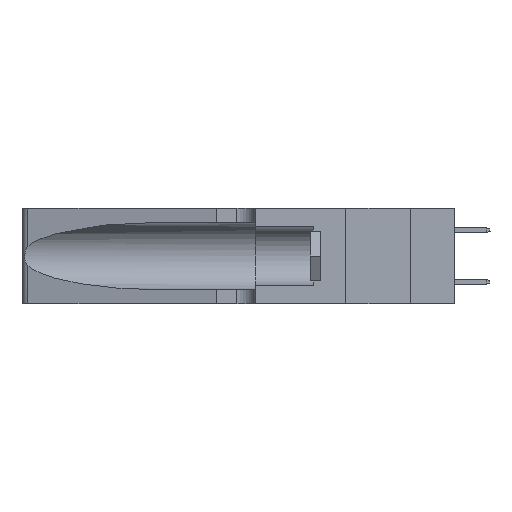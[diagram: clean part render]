
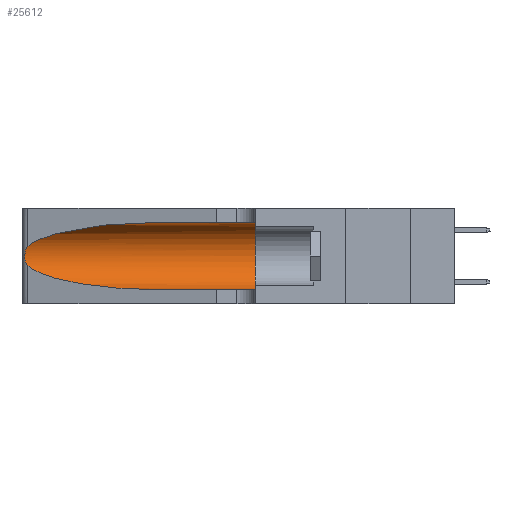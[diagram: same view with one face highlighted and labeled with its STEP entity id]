
A CAD part, left-side view. The second image highlights one B-rep face of the part: STEP entity #25612.
In plain terms, the highlighted cylindrical face has radius 3.308 mm (diameter 6.617 mm), a partial arc.
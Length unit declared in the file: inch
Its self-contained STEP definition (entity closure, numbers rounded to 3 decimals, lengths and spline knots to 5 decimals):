
#1521 = CARTESIAN_POINT ( 'NONE',  ( 0.26075, 1.23896, 0.19203 ) ) ;
#2905 = DIRECTION ( 'NONE',  ( 0., -1., 0. ) ) ;
#3774 = CARTESIAN_POINT ( 'NONE',  ( 0.25787, 1.23484, 0.2124 ) ) ;
#4326 = VERTEX_POINT ( 'NONE', #22807 ) ;
#4682 = CARTESIAN_POINT ( 'NONE',  ( 0.18966, 0.96281, 0.05475 ) ) ;
#4904 = CIRCLE ( 'NONE', #15176, 0.13025 ) ;
#5823 = VERTEX_POINT ( 'NONE', #24263 ) ;
#6220 = LINE ( 'NONE', #22452, #6288 ) ;
#6288 = VECTOR ( 'NONE', #8792, 39.37008 ) ;
#7240 = CYLINDRICAL_SURFACE ( 'NONE', #15799, 0.13025 ) ;
#7782 = B_SPLINE_CURVE_WITH_KNOTS ( 'NONE', 3,
 ( #24721, #13415, #13701, #3774, #8774, #27595, #1521, #20250, #27433, #15850, #29593, #20553, #20094, #10948 ),
 .UNSPECIFIED., .F., .F.,
 ( 4, 2, 2, 2, 2, 2, 4 ),
 ( 0., 0.00027, 0.00053, 0.00107, 0.0016, 0.00187, 0.00214 ),
 .UNSPECIFIED. ) ;
#8774 = CARTESIAN_POINT ( 'NONE',  ( 0.25854, 1.2359, 0.20912 ) ) ;
#8792 = DIRECTION ( 'NONE',  ( 0., -1., 0. ) ) ;
#9292 = CARTESIAN_POINT ( 'NONE',  ( 0.1305, 1.61858, 0.31525 ) ) ;
#9365 = CARTESIAN_POINT ( 'NONE',  ( 0.1305, 1.61858, 0.185 ) ) ;
#10886 =( BOUNDED_CURVE ( )  B_SPLINE_CURVE ( 3, ( #14642, #14173, #16597, #23944 ),
 .UNSPECIFIED., .F., .T. ) 
 B_SPLINE_CURVE_WITH_KNOTS ( ( 4, 4 ),
 ( 1.5708, 2.84003 ),
 .UNSPECIFIED. ) 
 CURVE ( )  GEOMETRIC_REPRESENTATION_ITEM ( )  RATIONAL_B_SPLINE_CURVE ( ( 1., 0.87, 0.87, 1. ) ) 
 REPRESENTATION_ITEM ( '' )  );
#10948 = CARTESIAN_POINT ( 'NONE',  ( 0.25487, 1.22718, 0.14631 ) ) ;
#11378 = EDGE_CURVE ( 'NONE', #4326, #26176, #6220, .T. ) ;
#11673 = FACE_OUTER_BOUND ( 'NONE', #22206, .T. ) ;
#11925 = EDGE_CURVE ( 'NONE', #13277, #26176, #4904, .T. ) ;
#12042 = CARTESIAN_POINT ( 'NONE',  ( 0.1305, 0.72297, 0.31525 ) ) ;
#12053 = LINE ( 'NONE', #9292, #14720 ) ;
#12310 = VERTEX_POINT ( 'NONE', #16334 ) ;
#12837 =( BOUNDED_CURVE ( )  B_SPLINE_CURVE ( 3, ( #13420, #25627, #4682, #14018 ),
 .UNSPECIFIED., .F., .T. ) 
 B_SPLINE_CURVE_WITH_KNOTS ( ( 4, 4 ),
 ( 3.44316, 4.71239 ),
 .UNSPECIFIED. ) 
 CURVE ( )  GEOMETRIC_REPRESENTATION_ITEM ( )  RATIONAL_B_SPLINE_CURVE ( ( 1., 0.87, 0.87, 1. ) ) 
 REPRESENTATION_ITEM ( '' )  );
#12985 = CARTESIAN_POINT ( 'NONE',  ( 0.1305, 0.35, 0.31525 ) ) ;
#13277 = VERTEX_POINT ( 'NONE', #12985 ) ;
#13415 = CARTESIAN_POINT ( 'NONE',  ( 0.25555, 1.22994, 0.2215 ) ) ;
#13420 = CARTESIAN_POINT ( 'NONE',  ( 0.25487, 1.22718, 0.14631 ) ) ;
#13436 = CARTESIAN_POINT ( 'NONE',  ( 0.1305, 0.35, 0.05475 ) ) ;
#13701 = CARTESIAN_POINT ( 'NONE',  ( 0.25639, 1.23184, 0.21858 ) ) ;
#14018 = CARTESIAN_POINT ( 'NONE',  ( 0.1305, 0.72297, 0.05475 ) ) ;
#14173 = CARTESIAN_POINT ( 'NONE',  ( 0.18966, 0.96281, 0.31525 ) ) ;
#14642 = CARTESIAN_POINT ( 'NONE',  ( 0.1305, 0.72297, 0.31525 ) ) ;
#14720 = VECTOR ( 'NONE', #2905, 39.37008 ) ;
#15176 = AXIS2_PLACEMENT_3D ( 'NONE', #24826, #27539, #15201 ) ;
#15201 = DIRECTION ( 'NONE',  ( 0., 0., 1. ) ) ;
#15799 = AXIS2_PLACEMENT_3D ( 'NONE', #9365, #25883, #20974 ) ;
#15850 = CARTESIAN_POINT ( 'NONE',  ( 0.25856, 1.23593, 0.16098 ) ) ;
#16172 = EDGE_CURVE ( 'NONE', #26030, #5823, #10886, .T. ) ;
#16334 = CARTESIAN_POINT ( 'NONE',  ( 0.25487, 1.22718, 0.14631 ) ) ;
#16597 = CARTESIAN_POINT ( 'NONE',  ( 0.2373, 1.15595, 0.28018 ) ) ;
#19498 = ORIENTED_EDGE ( 'NONE', *, *, #11925, .F. ) ;
#19509 = ORIENTED_EDGE ( 'NONE', *, *, #22715, .F. ) ;
#20094 = CARTESIAN_POINT ( 'NONE',  ( 0.25555, 1.22993, 0.14849 ) ) ;
#20250 = CARTESIAN_POINT ( 'NONE',  ( 0.26075, 1.23896, 0.178 ) ) ;
#20553 = CARTESIAN_POINT ( 'NONE',  ( 0.25639, 1.23186, 0.15144 ) ) ;
#20974 = DIRECTION ( 'NONE',  ( 0., 0., -1. ) ) ;
#21013 = EDGE_CURVE ( 'NONE', #5823, #12310, #7782, .T. ) ;
#22206 = EDGE_LOOP ( 'NONE', ( #23520, #28682, #24852, #24189, #19498, #19509 ) ) ;
#22452 = CARTESIAN_POINT ( 'NONE',  ( 0.1305, 1.61858, 0.05475 ) ) ;
#22715 = EDGE_CURVE ( 'NONE', #26030, #13277, #12053, .T. ) ;
#22807 = CARTESIAN_POINT ( 'NONE',  ( 0.1305, 0.72297, 0.05475 ) ) ;
#23520 = ORIENTED_EDGE ( 'NONE', *, *, #16172, .T. ) ;
#23801 = EDGE_CURVE ( 'NONE', #12310, #4326, #12837, .T. ) ;
#23944 = CARTESIAN_POINT ( 'NONE',  ( 0.25487, 1.22718, 0.22369 ) ) ;
#24189 = ORIENTED_EDGE ( 'NONE', *, *, #11378, .T. ) ;
#24263 = CARTESIAN_POINT ( 'NONE',  ( 0.25487, 1.22718, 0.22369 ) ) ;
#24721 = CARTESIAN_POINT ( 'NONE',  ( 0.25487, 1.22718, 0.22369 ) ) ;
#24826 = CARTESIAN_POINT ( 'NONE',  ( 0.1305, 0.35, 0.185 ) ) ;
#24852 = ORIENTED_EDGE ( 'NONE', *, *, #23801, .T. ) ;
#25612 = ADVANCED_FACE ( 'NONE', ( #11673 ), #7240, .F. ) ;
#25627 = CARTESIAN_POINT ( 'NONE',  ( 0.2373, 1.15595, 0.08982 ) ) ;
#25883 = DIRECTION ( 'NONE',  ( 0., -1., 0. ) ) ;
#26030 = VERTEX_POINT ( 'NONE', #12042 ) ;
#26176 = VERTEX_POINT ( 'NONE', #13436 ) ;
#27433 = CARTESIAN_POINT ( 'NONE',  ( 0.26017, 1.23833, 0.17102 ) ) ;
#27539 = DIRECTION ( 'NONE',  ( 0., 1., 0. ) ) ;
#27595 = CARTESIAN_POINT ( 'NONE',  ( 0.26018, 1.23835, 0.19895 ) ) ;
#28682 = ORIENTED_EDGE ( 'NONE', *, *, #21013, .T. ) ;
#29593 = CARTESIAN_POINT ( 'NONE',  ( 0.25789, 1.23486, 0.15765 ) ) ;
